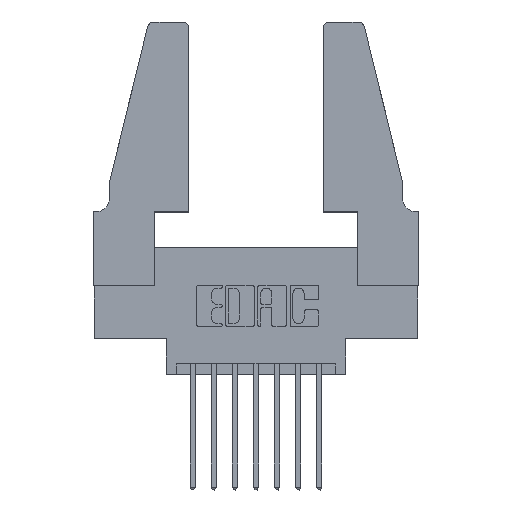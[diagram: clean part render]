
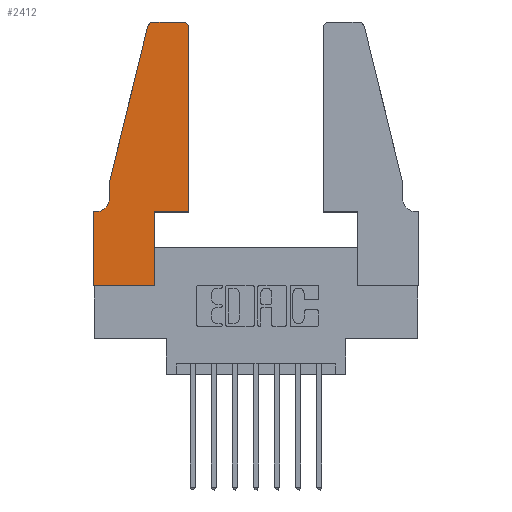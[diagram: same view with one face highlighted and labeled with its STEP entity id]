
A CAD part, top view. The second image highlights one B-rep face of the part: STEP entity #2412.
In plain terms, the highlighted planar face has unit normal (0, 0, 1).
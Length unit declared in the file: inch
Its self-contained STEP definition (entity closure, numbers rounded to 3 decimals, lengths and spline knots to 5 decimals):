
#249 = DIRECTION ( 'NONE',  ( 0., 0., 1. ) ) ;
#376 = CARTESIAN_POINT ( 'NONE',  ( 0.0755, 0.35, 0.37 ) ) ;
#735 = VECTOR ( 'NONE', #5475, 39.37008 ) ;
#812 = CARTESIAN_POINT ( 'NONE',  ( 0.0755, 0.42, 0.37 ) ) ;
#863 = ORIENTED_EDGE ( 'NONE', *, *, #6805, .T. ) ;
#868 = DIRECTION ( 'NONE',  ( 0., -1., 0. ) ) ;
#1013 = ORIENTED_EDGE ( 'NONE', *, *, #4511, .T. ) ;
#1027 = LINE ( 'NONE', #5472, #735 ) ;
#1103 = ORIENTED_EDGE ( 'NONE', *, *, #3661, .T. ) ;
#1112 = LINE ( 'NONE', #5290, #8535 ) ;
#1140 = VECTOR ( 'NONE', #11020, 39.37008 ) ;
#1173 = CARTESIAN_POINT ( 'NONE',  ( 0.4505, 1.22, 0.37 ) ) ;
#1174 = VERTEX_POINT ( 'NONE', #6863 ) ;
#1473 = DIRECTION ( 'NONE',  ( -0.239, -0.971, 0. ) ) ;
#1632 = AXIS2_PLACEMENT_3D ( 'NONE', #3058, #9790, #4036 ) ;
#1698 = CARTESIAN_POINT ( 'NONE',  ( 0.0055, 0.35, 0.37 ) ) ;
#1727 = EDGE_CURVE ( 'NONE', #2008, #1174, #11670, .T. ) ;
#2008 = VERTEX_POINT ( 'NONE', #5586 ) ;
#2064 = VERTEX_POINT ( 'NONE', #9965 ) ;
#2276 = ORIENTED_EDGE ( 'NONE', *, *, #11864, .T. ) ;
#2283 = VERTEX_POINT ( 'NONE', #1173 ) ;
#2350 = CARTESIAN_POINT ( 'NONE',  ( 0.4505, 0.35, 0.37 ) ) ;
#2412 = ADVANCED_FACE ( 'NONE', ( #9807 ), #11693, .T. ) ;
#2503 = DIRECTION ( 'NONE',  ( 0., -1., 0. ) ) ;
#2508 = VERTEX_POINT ( 'NONE', #10014 ) ;
#2529 = CARTESIAN_POINT ( 'NONE',  ( 0., 0., 0.37 ) ) ;
#2861 = VERTEX_POINT ( 'NONE', #11932 ) ;
#2917 = DIRECTION ( 'NONE',  ( 0., 0., 1. ) ) ;
#3058 = CARTESIAN_POINT ( 'NONE',  ( 0.0055, 0.42, 0.37 ) ) ;
#3308 = CARTESIAN_POINT ( 'NONE',  ( 0.4505, 0.35, 0.37 ) ) ;
#3661 = EDGE_CURVE ( 'NONE', #6003, #2508, #1027, .T. ) ;
#3967 = VECTOR ( 'NONE', #11607, 39.37008 ) ;
#4019 = LINE ( 'NONE', #3308, #1140 ) ;
#4020 = EDGE_CURVE ( 'NONE', #2861, #6003, #5288, .T. ) ;
#4036 = DIRECTION ( 'NONE',  ( -1., 0., 0. ) ) ;
#4419 = VECTOR ( 'NONE', #5200, 39.37008 ) ;
#4511 = EDGE_CURVE ( 'NONE', #4897, #8624, #4669, .T. ) ;
#4669 = LINE ( 'NONE', #7271, #7272 ) ;
#4843 = AXIS2_PLACEMENT_3D ( 'NONE', #6059, #249, #7049 ) ;
#4897 = VERTEX_POINT ( 'NONE', #7811 ) ;
#4910 = CIRCLE ( 'NONE', #4843, 0.03 ) ;
#5200 = DIRECTION ( 'NONE',  ( -1., 0., 0. ) ) ;
#5213 = ORIENTED_EDGE ( 'NONE', *, *, #6873, .T. ) ;
#5249 = DIRECTION ( 'NONE',  ( 0., 1., 0. ) ) ;
#5288 = LINE ( 'NONE', #2529, #10411 ) ;
#5290 = CARTESIAN_POINT ( 'NONE',  ( 0.4505, 0.35, 0.37 ) ) ;
#5350 = LINE ( 'NONE', #12435, #10172 ) ;
#5408 = EDGE_CURVE ( 'NONE', #2283, #2008, #8153, .T. ) ;
#5411 = AXIS2_PLACEMENT_3D ( 'NONE', #8710, #2917, #9656 ) ;
#5472 = CARTESIAN_POINT ( 'NONE',  ( 0., 0., 0.37 ) ) ;
#5475 = DIRECTION ( 'NONE',  ( 1., 0., 0. ) ) ;
#5586 = CARTESIAN_POINT ( 'NONE',  ( 0.4205, 1.25, 0.37 ) ) ;
#6003 = VERTEX_POINT ( 'NONE', #11487 ) ;
#6059 = CARTESIAN_POINT ( 'NONE',  ( 0.284, 1.22, 0.37 ) ) ;
#6397 = CARTESIAN_POINT ( 'NONE',  ( 0.0755, 0.5, 0.37 ) ) ;
#6445 = CARTESIAN_POINT ( 'NONE',  ( 0.2605, 1.25, 0.37 ) ) ;
#6805 = EDGE_CURVE ( 'NONE', #10728, #9591, #8121, .T. ) ;
#6863 = CARTESIAN_POINT ( 'NONE',  ( 0.284, 1.25, 0.37 ) ) ;
#6873 = EDGE_CURVE ( 'NONE', #1174, #4897, #4910, .T. ) ;
#6982 = EDGE_CURVE ( 'NONE', #2064, #10028, #4019, .T. ) ;
#7049 = DIRECTION ( 'NONE',  ( 1., 0., 0. ) ) ;
#7271 = CARTESIAN_POINT ( 'NONE',  ( 0.0755, 0.5, 0.37 ) ) ;
#7272 = VECTOR ( 'NONE', #1473, 39.37008 ) ;
#7339 = ORIENTED_EDGE ( 'NONE', *, *, #5408, .T. ) ;
#7612 = LINE ( 'NONE', #376, #4419 ) ;
#7811 = CARTESIAN_POINT ( 'NONE',  ( 0.25487, 1.22718, 0.37 ) ) ;
#7847 = ORIENTED_EDGE ( 'NONE', *, *, #1727, .T. ) ;
#8121 = CIRCLE ( 'NONE', #1632, 0.07 ) ;
#8153 = CIRCLE ( 'NONE', #5411, 0.03 ) ;
#8459 = DIRECTION ( 'NONE',  ( 0., 1., 0. ) ) ;
#8535 = VECTOR ( 'NONE', #5249, 39.37008 ) ;
#8624 = VERTEX_POINT ( 'NONE', #6397 ) ;
#8710 = CARTESIAN_POINT ( 'NONE',  ( 0.4205, 1.22, 0.37 ) ) ;
#8830 = VECTOR ( 'NONE', #8459, 39.37008 ) ;
#8873 = EDGE_CURVE ( 'NONE', #9591, #2861, #7612, .T. ) ;
#9129 = EDGE_LOOP ( 'NONE', ( #7847, #5213, #1013, #9370, #863, #12396, #11367, #1103, #2276, #11775, #12321, #7339 ) ) ;
#9370 = ORIENTED_EDGE ( 'NONE', *, *, #11954, .T. ) ;
#9591 = VERTEX_POINT ( 'NONE', #1698 ) ;
#9656 = DIRECTION ( 'NONE',  ( 1., 0., 0. ) ) ;
#9790 = DIRECTION ( 'NONE',  ( 0., 0., -1. ) ) ;
#9807 = FACE_OUTER_BOUND ( 'NONE', #9129, .T. ) ;
#9965 = CARTESIAN_POINT ( 'NONE',  ( 0.2865, 0.35, 0.37 ) ) ;
#10014 = CARTESIAN_POINT ( 'NONE',  ( 0.2865, 0., 0.37 ) ) ;
#10028 = VERTEX_POINT ( 'NONE', #2350 ) ;
#10172 = VECTOR ( 'NONE', #868, 39.37008 ) ;
#10411 = VECTOR ( 'NONE', #2503, 39.37008 ) ;
#10728 = VERTEX_POINT ( 'NONE', #812 ) ;
#11020 = DIRECTION ( 'NONE',  ( 1., 0., 0. ) ) ;
#11309 = CARTESIAN_POINT ( 'NONE',  ( 0.2865, 0.35, 0.37 ) ) ;
#11367 = ORIENTED_EDGE ( 'NONE', *, *, #4020, .T. ) ;
#11403 = LINE ( 'NONE', #11309, #8830 ) ;
#11487 = CARTESIAN_POINT ( 'NONE',  ( 0., 0., 0.37 ) ) ;
#11607 = DIRECTION ( 'NONE',  ( -1., 0., 0. ) ) ;
#11670 = LINE ( 'NONE', #6445, #3967 ) ;
#11693 = PLANE ( 'NONE',  #12342 ) ;
#11724 = DIRECTION ( 'NONE',  ( 1., 0., 0. ) ) ;
#11729 = DIRECTION ( 'NONE',  ( 0., 0., 1. ) ) ;
#11775 = ORIENTED_EDGE ( 'NONE', *, *, #6982, .T. ) ;
#11864 = EDGE_CURVE ( 'NONE', #2508, #2064, #11403, .T. ) ;
#11908 = CARTESIAN_POINT ( 'NONE',  ( 0., 0.35, 0.37 ) ) ;
#11932 = CARTESIAN_POINT ( 'NONE',  ( 0., 0.35, 0.37 ) ) ;
#11954 = EDGE_CURVE ( 'NONE', #8624, #10728, #5350, .T. ) ;
#12321 = ORIENTED_EDGE ( 'NONE', *, *, #12334, .T. ) ;
#12334 = EDGE_CURVE ( 'NONE', #10028, #2283, #1112, .T. ) ;
#12342 = AXIS2_PLACEMENT_3D ( 'NONE', #11908, #11729, #11724 ) ;
#12396 = ORIENTED_EDGE ( 'NONE', *, *, #8873, .T. ) ;
#12435 = CARTESIAN_POINT ( 'NONE',  ( 0.0755, 0.5, 0.37 ) ) ;
